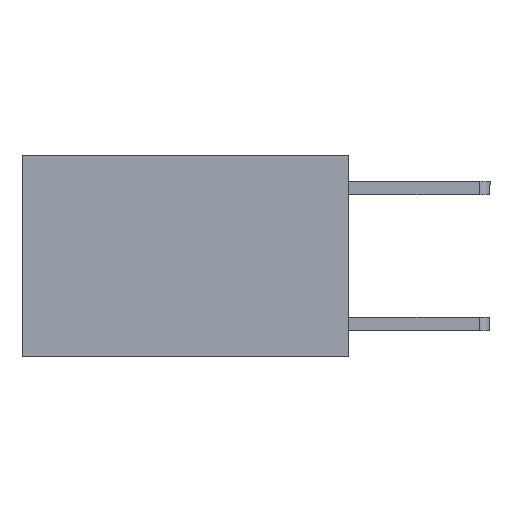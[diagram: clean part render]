
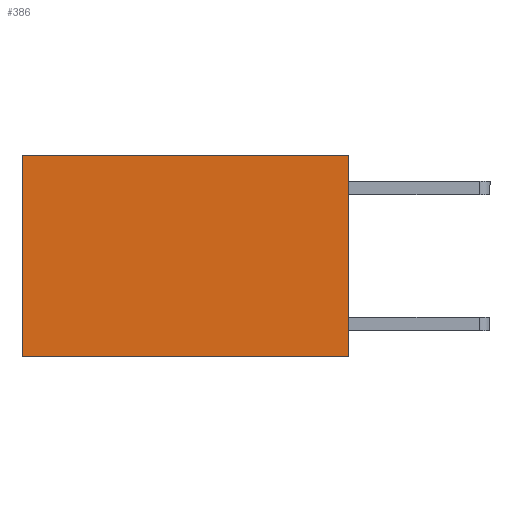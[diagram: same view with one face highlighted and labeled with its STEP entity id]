
A CAD part, left-side view. The second image highlights one B-rep face of the part: STEP entity #386.
In plain terms, the highlighted planar face has unit normal (-1, 0, 0).
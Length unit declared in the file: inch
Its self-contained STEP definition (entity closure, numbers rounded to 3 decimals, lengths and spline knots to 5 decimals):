
#292 = VERTEX_POINT ( 'NONE', #4434 ) ;
#386 = ADVANCED_FACE ( 'NONE', ( #455 ), #5519, .F. ) ;
#455 = FACE_OUTER_BOUND ( 'NONE', #10172, .T. ) ;
#564 = DIRECTION ( 'NONE',  ( 0., 0., -1. ) ) ;
#652 = VECTOR ( 'NONE', #9097, 39.37008 ) ;
#806 = ORIENTED_EDGE ( 'NONE', *, *, #896, .T. ) ;
#896 = EDGE_CURVE ( 'NONE', #3698, #6328, #9614, .T. ) ;
#930 = DIRECTION ( 'NONE',  ( 0., 1., 0. ) ) ;
#1338 = CARTESIAN_POINT ( 'NONE',  ( 0.2625, 0.6, 0. ) ) ;
#2636 = CARTESIAN_POINT ( 'NONE',  ( 0.2625, 0., 0. ) ) ;
#2749 = EDGE_CURVE ( 'NONE', #3700, #3698, #7693, .T. ) ;
#2792 = CARTESIAN_POINT ( 'NONE',  ( 0.2625, 0., 0. ) ) ;
#2978 = DIRECTION ( 'NONE',  ( 1., 0., 0. ) ) ;
#3588 = ORIENTED_EDGE ( 'NONE', *, *, #8512, .F. ) ;
#3698 = VERTEX_POINT ( 'NONE', #9954 ) ;
#3700 = VERTEX_POINT ( 'NONE', #2636 ) ;
#4330 = DIRECTION ( 'NONE',  ( 0., 1., 0. ) ) ;
#4408 = LINE ( 'NONE', #2792, #652 ) ;
#4416 = VECTOR ( 'NONE', #930, 39.37008 ) ;
#4434 = CARTESIAN_POINT ( 'NONE',  ( 0.2625, 0., -0.37 ) ) ;
#5116 = EDGE_CURVE ( 'NONE', #3700, #292, #4408, .T. ) ;
#5140 = VECTOR ( 'NONE', #4330, 39.37008 ) ;
#5249 = CARTESIAN_POINT ( 'NONE',  ( 0.2625, 0., 0. ) ) ;
#5519 = PLANE ( 'NONE',  #9639 ) ;
#6206 = ORIENTED_EDGE ( 'NONE', *, *, #2749, .T. ) ;
#6328 = VERTEX_POINT ( 'NONE', #9045 ) ;
#6662 = CARTESIAN_POINT ( 'NONE',  ( 0.2625, 0., -0.37 ) ) ;
#7693 = LINE ( 'NONE', #5249, #5140 ) ;
#7775 = ORIENTED_EDGE ( 'NONE', *, *, #5116, .F. ) ;
#8512 = EDGE_CURVE ( 'NONE', #292, #6328, #8917, .T. ) ;
#8917 = LINE ( 'NONE', #6662, #4416 ) ;
#8988 = VECTOR ( 'NONE', #10374, 39.37008 ) ;
#9045 = CARTESIAN_POINT ( 'NONE',  ( 0.2625, 0.6, -0.37 ) ) ;
#9097 = DIRECTION ( 'NONE',  ( 0., 0., -1. ) ) ;
#9388 = CARTESIAN_POINT ( 'NONE',  ( 0.2625, 0., 0. ) ) ;
#9614 = LINE ( 'NONE', #1338, #8988 ) ;
#9639 = AXIS2_PLACEMENT_3D ( 'NONE', #9388, #2978, #564 ) ;
#9954 = CARTESIAN_POINT ( 'NONE',  ( 0.2625, 0.6, 0. ) ) ;
#10172 = EDGE_LOOP ( 'NONE', ( #806, #3588, #7775, #6206 ) ) ;
#10374 = DIRECTION ( 'NONE',  ( 0., 0., -1. ) ) ;
